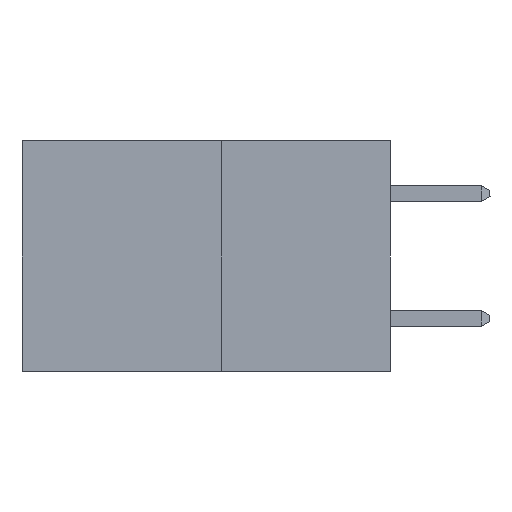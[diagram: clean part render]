
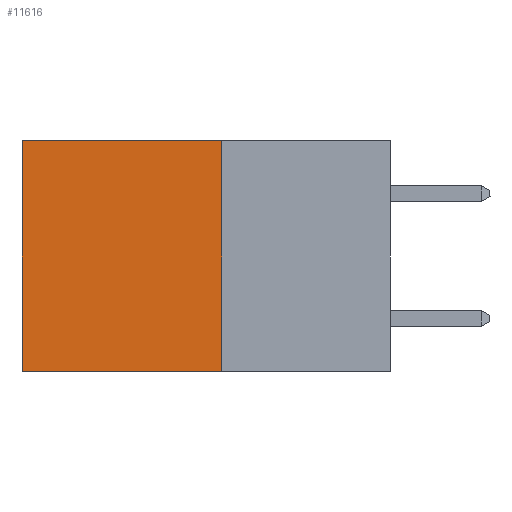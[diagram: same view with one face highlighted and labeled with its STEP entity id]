
A CAD part, left-side view. The second image highlights one B-rep face of the part: STEP entity #11616.
In plain terms, the highlighted planar face has unit normal (-1, 0, 0).
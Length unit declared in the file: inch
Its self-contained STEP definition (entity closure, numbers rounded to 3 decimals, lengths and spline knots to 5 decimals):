
#501 = VERTEX_POINT ( 'NONE', #2878 ) ;
#888 = EDGE_CURVE ( 'NONE', #6317, #501, #9200, .T. ) ;
#1769 = AXIS2_PLACEMENT_3D ( 'NONE', #4391, #20199, #8445 ) ;
#2423 = PLANE ( 'NONE',  #1769 ) ;
#2878 = CARTESIAN_POINT ( 'NONE',  ( 0.277, 0.59, 0. ) ) ;
#3135 = ORIENTED_EDGE ( 'NONE', *, *, #21775, .T. ) ;
#3972 = CARTESIAN_POINT ( 'NONE',  ( 0.277, 0.27, -0.37 ) ) ;
#4391 = CARTESIAN_POINT ( 'NONE',  ( 0.277, 0.27, -0.37 ) ) ;
#4460 = EDGE_LOOP ( 'NONE', ( #3135, #23001, #18879, #11350 ) ) ;
#6317 = VERTEX_POINT ( 'NONE', #14556 ) ;
#6510 = LINE ( 'NONE', #3972, #11757 ) ;
#8445 = DIRECTION ( 'NONE',  ( 0., 0., -1. ) ) ;
#8604 = FACE_OUTER_BOUND ( 'NONE', #4460, .T. ) ;
#9200 = LINE ( 'NONE', #17909, #19031 ) ;
#9474 = EDGE_CURVE ( 'NONE', #24467, #11025, #6510, .T. ) ;
#10487 = CARTESIAN_POINT ( 'NONE',  ( 0.277, 0.59, -0.37 ) ) ;
#11025 = VERTEX_POINT ( 'NONE', #10487 ) ;
#11350 = ORIENTED_EDGE ( 'NONE', *, *, #888, .T. ) ;
#11616 = ADVANCED_FACE ( 'NONE', ( #8604 ), #2423, .F. ) ;
#11757 = VECTOR ( 'NONE', #17752, 39.37008 ) ;
#12759 = VECTOR ( 'NONE', #13851, 39.37008 ) ;
#12775 = CARTESIAN_POINT ( 'NONE',  ( 0.277, 0.27, -0.37 ) ) ;
#13851 = DIRECTION ( 'NONE',  ( 0., 0., -1. ) ) ;
#14191 = VECTOR ( 'NONE', #14691, 39.37008 ) ;
#14556 = CARTESIAN_POINT ( 'NONE',  ( 0.277, 0.27, 0. ) ) ;
#14691 = DIRECTION ( 'NONE',  ( 0., 0., -1. ) ) ;
#16058 = CARTESIAN_POINT ( 'NONE',  ( 0.277, 0.27, -0.37 ) ) ;
#17752 = DIRECTION ( 'NONE',  ( 0., 1., 0. ) ) ;
#17909 = CARTESIAN_POINT ( 'NONE',  ( 0.277, 0.27, 0. ) ) ;
#18879 = ORIENTED_EDGE ( 'NONE', *, *, #24704, .F. ) ;
#19031 = VECTOR ( 'NONE', #24329, 39.37008 ) ;
#19694 = CARTESIAN_POINT ( 'NONE',  ( 0.277, 0.59, -0.37 ) ) ;
#20199 = DIRECTION ( 'NONE',  ( 1., 0., 0. ) ) ;
#21775 = EDGE_CURVE ( 'NONE', #501, #11025, #23727, .T. ) ;
#23001 = ORIENTED_EDGE ( 'NONE', *, *, #9474, .F. ) ;
#23727 = LINE ( 'NONE', #19694, #12759 ) ;
#24329 = DIRECTION ( 'NONE',  ( 0., 1., 0. ) ) ;
#24467 = VERTEX_POINT ( 'NONE', #16058 ) ;
#24474 = LINE ( 'NONE', #12775, #14191 ) ;
#24704 = EDGE_CURVE ( 'NONE', #6317, #24467, #24474, .T. ) ;
